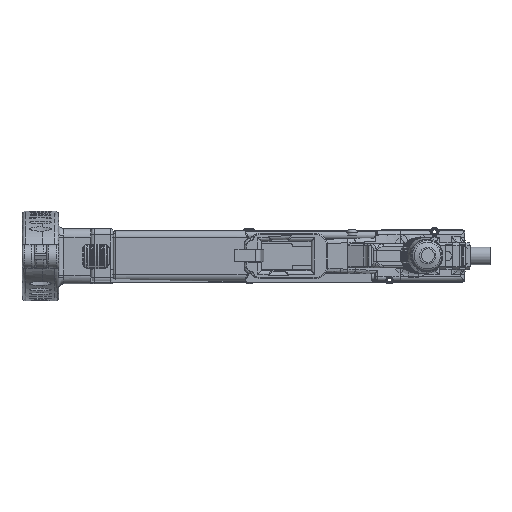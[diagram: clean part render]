
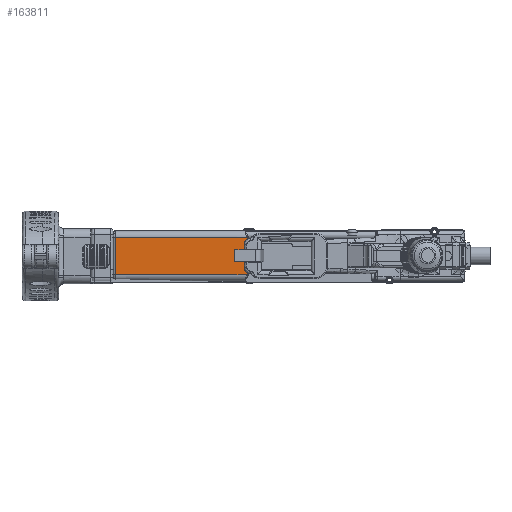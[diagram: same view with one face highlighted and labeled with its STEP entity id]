
A CAD part, front view. The second image highlights one B-rep face of the part: STEP entity #163811.
In plain terms, the highlighted planar face has unit normal (-0.038, -0.999, 0).
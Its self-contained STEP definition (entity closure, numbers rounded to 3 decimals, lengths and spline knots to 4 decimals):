
#6531=B_SPLINE_CURVE_WITH_KNOTS('',3,(#341526,#341527,#341528,#341529,#341530,
#341531),.UNSPECIFIED.,.F.,.F.,(4,2,4),(2.3604,2.488,
2.5839),.UNSPECIFIED.);
#6532=B_SPLINE_CURVE_WITH_KNOTS('',3,(#341532,#341533,#341534,#341535,#341536,
#341537),.UNSPECIFIED.,.F.,.F.,(4,2,4),(2.5839,2.6797,
2.7899),.UNSPECIFIED.);
#23175=FACE_OUTER_BOUND('',#33211,.T.);
#33211=EDGE_LOOP('',(#116834,#116835,#116836,#116837,#116838,#116839,#116840,
#116841));
#44548=LINE('',#340992,#56102);
#44563=LINE('',#341466,#56117);
#44564=LINE('',#341518,#56118);
#44565=LINE('',#341522,#56119);
#44566=LINE('',#341524,#56120);
#44567=LINE('',#341525,#56121);
#56102=VECTOR('',#196968,0.3937);
#56117=VECTOR('',#197013,0.3937);
#56118=VECTOR('',#197020,0.3937);
#56119=VECTOR('',#197023,0.3937);
#56120=VECTOR('',#197024,0.3937);
#56121=VECTOR('',#197025,0.3937);
#68266=VERTEX_POINT('',#340988);
#68267=VERTEX_POINT('',#340990);
#68290=VERTEX_POINT('',#341463);
#68291=VERTEX_POINT('',#341465);
#68292=VERTEX_POINT('',#341503);
#68293=VERTEX_POINT('',#341520);
#68294=VERTEX_POINT('',#341521);
#68295=VERTEX_POINT('',#341523);
#86269=EDGE_CURVE('',#68266,#68267,#44548,.T.);
#86302=EDGE_CURVE('',#68290,#68291,#44563,.T.);
#86307=EDGE_CURVE('',#68292,#68290,#44564,.T.);
#86308=EDGE_CURVE('',#68293,#68294,#44565,.T.);
#86309=EDGE_CURVE('',#68295,#68293,#44566,.T.);
#86310=EDGE_CURVE('',#68291,#68295,#44567,.T.);
#86311=EDGE_CURVE('',#68292,#68266,#6531,.T.);
#86312=EDGE_CURVE('',#68267,#68294,#6532,.T.);
#116834=ORIENTED_EDGE('',*,*,#86308,.F.);
#116835=ORIENTED_EDGE('',*,*,#86309,.F.);
#116836=ORIENTED_EDGE('',*,*,#86310,.F.);
#116837=ORIENTED_EDGE('',*,*,#86302,.F.);
#116838=ORIENTED_EDGE('',*,*,#86307,.F.);
#116839=ORIENTED_EDGE('',*,*,#86311,.T.);
#116840=ORIENTED_EDGE('',*,*,#86269,.T.);
#116841=ORIENTED_EDGE('',*,*,#86312,.T.);
#159225=PLANE('',#174964);
#163811=ADVANCED_FACE('',(#23175),#159225,.F.);
#174964=AXIS2_PLACEMENT_3D('',#341519,#197021,#197022);
#196968=DIRECTION('',(0.,0.,1.));
#197013=DIRECTION('',(-0.999,0.038,0.));
#197020=DIRECTION('',(-0.505,0.019,-0.863));
#197021=DIRECTION('center_axis',(0.038,0.999,0.));
#197022=DIRECTION('ref_axis',(0.999,-0.038,0.));
#197023=DIRECTION('',(0.497,-0.019,-0.868));
#197024=DIRECTION('',(0.999,-0.038,0.));
#197025=DIRECTION('',(0.,0.,1.));
#340988=CARTESIAN_POINT('',(-5.2169,-1.0034,0.33));
#340990=CARTESIAN_POINT('',(-5.2169,-1.0034,0.835));
#340992=CARTESIAN_POINT('',(-5.2169,-1.0034,0.5825));
#341463=CARTESIAN_POINT('',(-5.3277,-0.9991,-0.0031));
#341465=CARTESIAN_POINT('',(-9.4273,-0.8414,-0.0031));
#341466=CARTESIAN_POINT('',(-8.7128,-0.8688,-0.0031));
#341503=CARTESIAN_POINT('',(-5.1825,-1.0047,0.2448));
#341518=CARTESIAN_POINT('',(-5.5452,-0.9907,-0.3747));
#341519=CARTESIAN_POINT('Origin',(-9.262,-0.8477,
1.365));
#341520=CARTESIAN_POINT('',(-5.3319,-0.9989,1.1681));
#341521=CARTESIAN_POINT('',(-5.1866,-1.0045,0.9145));
#341522=CARTESIAN_POINT('',(-5.9025,-0.977,2.164));
#341523=CARTESIAN_POINT('',(-9.4273,-0.8414,1.1681));
#341524=CARTESIAN_POINT('',(-4.4921,-1.0312,1.1681));
#341525=CARTESIAN_POINT('',(-9.4273,-0.8414,0.9738));
#341526=CARTESIAN_POINT('Ctrl Pts',(-5.1825,-1.0047,
0.2448));
#341527=CARTESIAN_POINT('Ctrl Pts',(-5.1925,-1.0043,
0.2583));
#341528=CARTESIAN_POINT('Ctrl Pts',(-5.203,-1.0039,
0.2754));
#341529=CARTESIAN_POINT('Ctrl Pts',(-5.2137,-1.0035,
0.3027));
#341530=CARTESIAN_POINT('Ctrl Pts',(-5.2169,-1.0034,
0.3174));
#341531=CARTESIAN_POINT('Ctrl Pts',(-5.2169,-1.0034,
0.33));
#341532=CARTESIAN_POINT('Ctrl Pts',(-5.2169,-1.0034,
0.835));
#341533=CARTESIAN_POINT('Ctrl Pts',(-5.2169,-1.0034,
0.8476));
#341534=CARTESIAN_POINT('Ctrl Pts',(-5.2137,-1.0035,
0.8623));
#341535=CARTESIAN_POINT('Ctrl Pts',(-5.2039,-1.0039,
0.8875));
#341536=CARTESIAN_POINT('Ctrl Pts',(-5.1953,-1.0042,
0.9021));
#341537=CARTESIAN_POINT('Ctrl Pts',(-5.1866,-1.0045,
0.9145));
